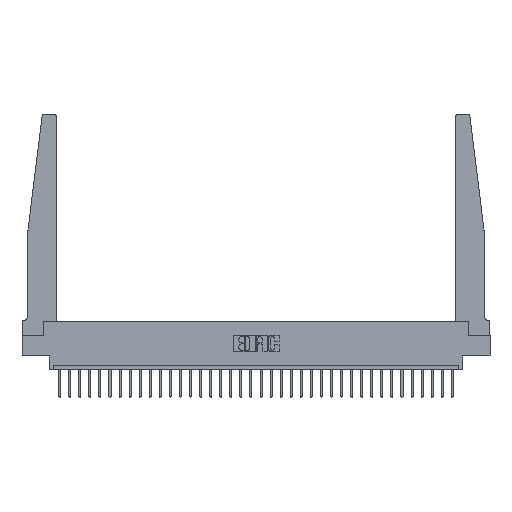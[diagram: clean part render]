
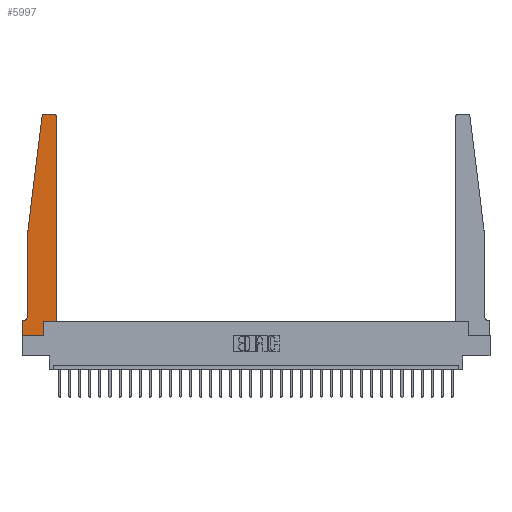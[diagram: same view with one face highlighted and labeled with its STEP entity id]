
A CAD part, top view. The second image highlights one B-rep face of the part: STEP entity #5997.
In plain terms, the highlighted planar face has unit normal (0, 0, 1).
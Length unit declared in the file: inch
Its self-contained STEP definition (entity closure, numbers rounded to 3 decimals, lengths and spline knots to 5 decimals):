
#13 = VERTEX_POINT ( 'NONE', #4900 ) ;
#191 = CARTESIAN_POINT ( 'NONE',  ( 0., 0., 0.37 ) ) ;
#345 = EDGE_CURVE ( 'NONE', #16499, #29626, #14343, .T. ) ;
#410 = EDGE_CURVE ( 'NONE', #29626, #9511, #12197, .T. ) ;
#992 = CARTESIAN_POINT ( 'NONE',  ( 0.395, 2.72, 0.37 ) ) ;
#1158 = DIRECTION ( 'NONE',  ( 0., 1., 0. ) ) ;
#1650 = CARTESIAN_POINT ( 'NONE',  ( 0., 0.1875, 0.37 ) ) ;
#2112 = VECTOR ( 'NONE', #1158, 39.37008 ) ;
#2917 = AXIS2_PLACEMENT_3D ( 'NONE', #992, #17867, #26394 ) ;
#3083 = ORIENTED_EDGE ( 'NONE', *, *, #345, .T. ) ;
#3530 = LINE ( 'NONE', #8864, #12867 ) ;
#3609 = CARTESIAN_POINT ( 'NONE',  ( 0.2605, 0.18, 0.37 ) ) ;
#4344 = LINE ( 'NONE', #29371, #13685 ) ;
#4403 = VECTOR ( 'NONE', #13651, 39.37008 ) ;
#4659 = DIRECTION ( 'NONE',  ( 0., -1., 0. ) ) ;
#4900 = CARTESIAN_POINT ( 'NONE',  ( 0.425, 0.18, 0.37 ) ) ;
#4948 = CARTESIAN_POINT ( 'NONE',  ( 0.065, 1.25, 0.37 ) ) ;
#5320 = VERTEX_POINT ( 'NONE', #6588 ) ;
#5504 = CARTESIAN_POINT ( 'NONE',  ( 0.065, 1.25, 0.37 ) ) ;
#5526 = LINE ( 'NONE', #191, #23943 ) ;
#5997 = ADVANCED_FACE ( 'NONE', ( #13232 ), #18324, .T. ) ;
#6016 = EDGE_CURVE ( 'NONE', #10415, #6760, #5526, .T. ) ;
#6550 = AXIS2_PLACEMENT_3D ( 'NONE', #14617, #24098, #29631 ) ;
#6588 = CARTESIAN_POINT ( 'NONE',  ( 0.065, 0.2375, 0.37 ) ) ;
#6724 = EDGE_CURVE ( 'NONE', #6760, #7691, #8278, .T. ) ;
#6760 = VERTEX_POINT ( 'NONE', #29000 ) ;
#7097 = ORIENTED_EDGE ( 'NONE', *, *, #9378, .T. ) ;
#7691 = VERTEX_POINT ( 'NONE', #24358 ) ;
#8278 = LINE ( 'NONE', #3609, #2112 ) ;
#8475 = VERTEX_POINT ( 'NONE', #27223 ) ;
#8864 = CARTESIAN_POINT ( 'NONE',  ( 0.425, 0.18, 0.37 ) ) ;
#8929 = DIRECTION ( 'NONE',  ( 0., 1., 0. ) ) ;
#9207 = EDGE_CURVE ( 'NONE', #9511, #5320, #12050, .T. ) ;
#9378 = EDGE_CURVE ( 'NONE', #5320, #10832, #16691, .T. ) ;
#9430 = CARTESIAN_POINT ( 'NONE',  ( 0., 0., 0.37 ) ) ;
#9511 = VERTEX_POINT ( 'NONE', #5504 ) ;
#10058 = EDGE_CURVE ( 'NONE', #24393, #10415, #21065, .T. ) ;
#10415 = VERTEX_POINT ( 'NONE', #28921 ) ;
#10457 = ORIENTED_EDGE ( 'NONE', *, *, #410, .T. ) ;
#10832 = VERTEX_POINT ( 'NONE', #21863 ) ;
#10903 = ORIENTED_EDGE ( 'NONE', *, *, #12149, .T. ) ;
#11123 = DIRECTION ( 'NONE',  ( 0., 0., 1. ) ) ;
#12008 = DIRECTION ( 'NONE',  ( 1., 0., 0. ) ) ;
#12050 = LINE ( 'NONE', #28249, #22920 ) ;
#12149 = EDGE_CURVE ( 'NONE', #7691, #13, #3530, .T. ) ;
#12197 = LINE ( 'NONE', #4948, #23450 ) ;
#12627 = ORIENTED_EDGE ( 'NONE', *, *, #6016, .T. ) ;
#12867 = VECTOR ( 'NONE', #24856, 39.37008 ) ;
#13232 = FACE_OUTER_BOUND ( 'NONE', #22696, .T. ) ;
#13651 = DIRECTION ( 'NONE',  ( -1., 0., 0. ) ) ;
#13685 = VECTOR ( 'NONE', #18071, 39.37008 ) ;
#13738 = LINE ( 'NONE', #27776, #4403 ) ;
#13923 = DIRECTION ( 'NONE',  ( 0., -1., 0. ) ) ;
#14343 = CIRCLE ( 'NONE', #20050, 0.03 ) ;
#14617 = CARTESIAN_POINT ( 'NONE',  ( 0.015, 0.2375, 0.37 ) ) ;
#14619 = AXIS2_PLACEMENT_3D ( 'NONE', #25455, #11123, #23347 ) ;
#15027 = EDGE_CURVE ( 'NONE', #17857, #16499, #13738, .T. ) ;
#15606 = EDGE_CURVE ( 'NONE', #10832, #24393, #4344, .T. ) ;
#15676 = EDGE_CURVE ( 'NONE', #13, #8475, #28972, .T. ) ;
#15729 = DIRECTION ( 'NONE',  ( 0., 0., 1. ) ) ;
#15779 = ORIENTED_EDGE ( 'NONE', *, *, #10058, .T. ) ;
#16499 = VERTEX_POINT ( 'NONE', #24684 ) ;
#16691 = CIRCLE ( 'NONE', #6550, 0.05 ) ;
#16930 = ORIENTED_EDGE ( 'NONE', *, *, #15606, .T. ) ;
#17857 = VERTEX_POINT ( 'NONE', #24936 ) ;
#17867 = DIRECTION ( 'NONE',  ( 0., 0., 1. ) ) ;
#18071 = DIRECTION ( 'NONE',  ( -1., 0., 0. ) ) ;
#18074 = DIRECTION ( 'NONE',  ( 1., 0., 0. ) ) ;
#18324 = PLANE ( 'NONE',  #14619 ) ;
#19439 = ORIENTED_EDGE ( 'NONE', *, *, #6724, .T. ) ;
#20000 = EDGE_CURVE ( 'NONE', #8475, #17857, #27435, .T. ) ;
#20050 = AXIS2_PLACEMENT_3D ( 'NONE', #27317, #15729, #18074 ) ;
#20413 = ORIENTED_EDGE ( 'NONE', *, *, #9207, .T. ) ;
#21065 = LINE ( 'NONE', #9430, #25104 ) ;
#21863 = CARTESIAN_POINT ( 'NONE',  ( 0.015, 0.1875, 0.37 ) ) ;
#22007 = ORIENTED_EDGE ( 'NONE', *, *, #20000, .T. ) ;
#22696 = EDGE_LOOP ( 'NONE', ( #23925, #3083, #10457, #20413, #7097, #16930, #15779, #12627, #19439, #10903, #28916, #22007 ) ) ;
#22920 = VECTOR ( 'NONE', #13923, 39.37008 ) ;
#23152 = DIRECTION ( 'NONE',  ( -0.122, -0.992, 0. ) ) ;
#23347 = DIRECTION ( 'NONE',  ( 1., 0., 0. ) ) ;
#23450 = VECTOR ( 'NONE', #23152, 39.37008 ) ;
#23925 = ORIENTED_EDGE ( 'NONE', *, *, #15027, .T. ) ;
#23943 = VECTOR ( 'NONE', #12008, 39.37008 ) ;
#24098 = DIRECTION ( 'NONE',  ( 0., 0., -1. ) ) ;
#24358 = CARTESIAN_POINT ( 'NONE',  ( 0.2605, 0.18, 0.37 ) ) ;
#24393 = VERTEX_POINT ( 'NONE', #1650 ) ;
#24654 = CARTESIAN_POINT ( 'NONE',  ( 0.24675, 2.72367, 0.37 ) ) ;
#24684 = CARTESIAN_POINT ( 'NONE',  ( 0.27653, 2.75, 0.37 ) ) ;
#24693 = CARTESIAN_POINT ( 'NONE',  ( 0.425, 0.18, 0.37 ) ) ;
#24856 = DIRECTION ( 'NONE',  ( 1., 0., 0. ) ) ;
#24936 = CARTESIAN_POINT ( 'NONE',  ( 0.395, 2.75, 0.37 ) ) ;
#24993 = VECTOR ( 'NONE', #8929, 39.37008 ) ;
#25104 = VECTOR ( 'NONE', #4659, 39.37008 ) ;
#25455 = CARTESIAN_POINT ( 'NONE',  ( 0., 0.1875, 0.37 ) ) ;
#26394 = DIRECTION ( 'NONE',  ( 1., 0., 0. ) ) ;
#27223 = CARTESIAN_POINT ( 'NONE',  ( 0.425, 2.72, 0.37 ) ) ;
#27317 = CARTESIAN_POINT ( 'NONE',  ( 0.27653, 2.72, 0.37 ) ) ;
#27435 = CIRCLE ( 'NONE', #2917, 0.03 ) ;
#27776 = CARTESIAN_POINT ( 'NONE',  ( 0.25, 2.75, 0.37 ) ) ;
#28249 = CARTESIAN_POINT ( 'NONE',  ( 0.065, 1.25, 0.37 ) ) ;
#28916 = ORIENTED_EDGE ( 'NONE', *, *, #15676, .T. ) ;
#28921 = CARTESIAN_POINT ( 'NONE',  ( 0., 0., 0.37 ) ) ;
#28972 = LINE ( 'NONE', #24693, #24993 ) ;
#29000 = CARTESIAN_POINT ( 'NONE',  ( 0.2605, 0., 0.37 ) ) ;
#29371 = CARTESIAN_POINT ( 'NONE',  ( 0.065, 0.1875, 0.37 ) ) ;
#29626 = VERTEX_POINT ( 'NONE', #24654 ) ;
#29631 = DIRECTION ( 'NONE',  ( -1., 0., 0. ) ) ;
